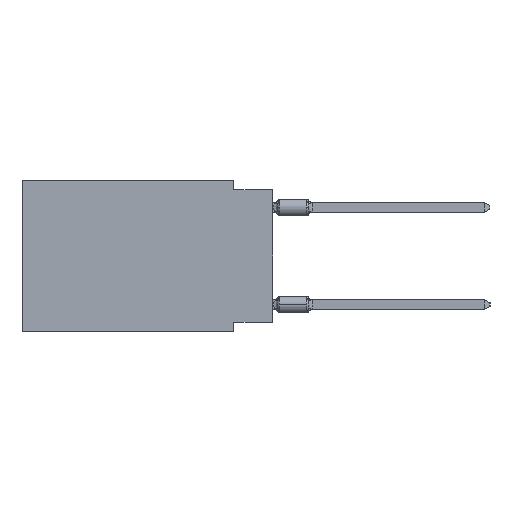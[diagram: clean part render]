
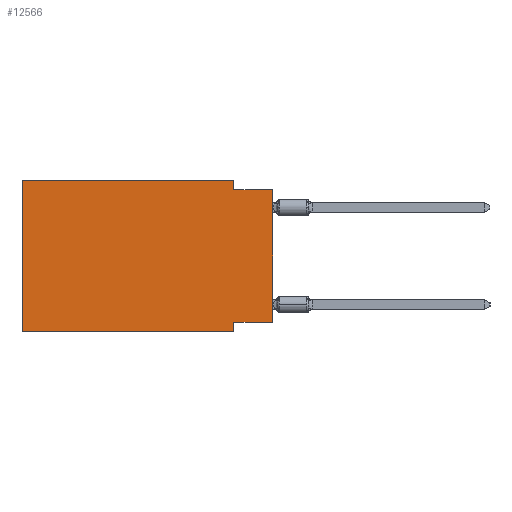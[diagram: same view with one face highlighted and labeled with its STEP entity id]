
A CAD part, left-side view. The second image highlights one B-rep face of the part: STEP entity #12566.
In plain terms, the highlighted planar face has unit normal (-1, 0, 0).
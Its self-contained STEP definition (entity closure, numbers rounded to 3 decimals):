
#699 = DIRECTION ( 'NONE',  ( 0., 0., 1. ) ) ;
#1057 = LINE ( 'NONE', #15567, #5075 ) ;
#2091 = CARTESIAN_POINT ( 'NONE',  ( 0., 2.54, -9.906 ) ) ;
#2407 = DIRECTION ( 'NONE',  ( 1., 0., 0. ) ) ;
#2442 = EDGE_CURVE ( 'NONE', #17567, #22266, #21646, .T. ) ;
#2515 = DIRECTION ( 'NONE',  ( 0., -1., 0. ) ) ;
#2831 = ORIENTED_EDGE ( 'NONE', *, *, #2442, .F. ) ;
#3285 = EDGE_LOOP ( 'NONE', ( #28138, #15857, #26342, #2831, #25457, #26435, #29695, #28562 ) ) ;
#3468 = VECTOR ( 'NONE', #11607, 1000. ) ;
#3684 = CARTESIAN_POINT ( 'NONE',  ( 0., 16.383, -9.906 ) ) ;
#4875 = FACE_OUTER_BOUND ( 'NONE', #3285, .T. ) ;
#5047 = PLANE ( 'NONE',  #10372 ) ;
#5075 = VECTOR ( 'NONE', #17880, 1000. ) ;
#5175 = CARTESIAN_POINT ( 'NONE',  ( 0., 16.383, 0. ) ) ;
#5462 = CARTESIAN_POINT ( 'NONE',  ( 0., 2.54, 0. ) ) ;
#6109 = LINE ( 'NONE', #26071, #17773 ) ;
#6618 = VERTEX_POINT ( 'NONE', #10996 ) ;
#6653 = CARTESIAN_POINT ( 'NONE',  ( 0., 0., 0. ) ) ;
#8192 = VECTOR ( 'NONE', #22129, 1000. ) ;
#8755 = VECTOR ( 'NONE', #25015, 1000. ) ;
#8970 = EDGE_CURVE ( 'NONE', #23673, #24792, #15040, .T. ) ;
#9190 = CARTESIAN_POINT ( 'NONE',  ( 0., 16.383, -9.906 ) ) ;
#9498 = VECTOR ( 'NONE', #2515, 1000. ) ;
#10372 = AXIS2_PLACEMENT_3D ( 'NONE', #29936, #2407, #15100 ) ;
#10996 = CARTESIAN_POINT ( 'NONE',  ( 0., 2.54, -9.271 ) ) ;
#11607 = DIRECTION ( 'NONE',  ( 0., 0., 1. ) ) ;
#12566 = ADVANCED_FACE ( 'NONE', ( #4875 ), #5047, .F. ) ;
#12947 = CARTESIAN_POINT ( 'NONE',  ( 0., 2.54, -0.635 ) ) ;
#13725 = EDGE_CURVE ( 'NONE', #6618, #31249, #6109, .T. ) ;
#15040 = LINE ( 'NONE', #25112, #9498 ) ;
#15100 = DIRECTION ( 'NONE',  ( 0., 0., -1. ) ) ;
#15471 = VERTEX_POINT ( 'NONE', #21390 ) ;
#15567 = CARTESIAN_POINT ( 'NONE',  ( 0., 2.54, 0. ) ) ;
#15857 = ORIENTED_EDGE ( 'NONE', *, *, #8970, .F. ) ;
#17340 = CARTESIAN_POINT ( 'NONE',  ( 0., 0., -0.635 ) ) ;
#17414 = CARTESIAN_POINT ( 'NONE',  ( 0., 0., -9.271 ) ) ;
#17567 = VERTEX_POINT ( 'NONE', #22792 ) ;
#17574 = LINE ( 'NONE', #17414, #8755 ) ;
#17773 = VECTOR ( 'NONE', #18135, 1000. ) ;
#17880 = DIRECTION ( 'NONE',  ( 0., 0., -1. ) ) ;
#18135 = DIRECTION ( 'NONE',  ( 0., 0., -1. ) ) ;
#18755 = LINE ( 'NONE', #9190, #25879 ) ;
#20800 = LINE ( 'NONE', #5175, #28158 ) ;
#21390 = CARTESIAN_POINT ( 'NONE',  ( 0., 0., -9.271 ) ) ;
#21646 = LINE ( 'NONE', #24619, #8192 ) ;
#21679 = EDGE_CURVE ( 'NONE', #30647, #31249, #18755, .T. ) ;
#21799 = LINE ( 'NONE', #6653, #3468 ) ;
#22129 = DIRECTION ( 'NONE',  ( 0., -1., 0. ) ) ;
#22266 = VERTEX_POINT ( 'NONE', #5462 ) ;
#22792 = CARTESIAN_POINT ( 'NONE',  ( 0., 16.383, 0. ) ) ;
#23629 = EDGE_CURVE ( 'NONE', #22266, #23673, #1057, .T. ) ;
#23673 = VERTEX_POINT ( 'NONE', #12947 ) ;
#23806 = EDGE_CURVE ( 'NONE', #15471, #24792, #21799, .T. ) ;
#24619 = CARTESIAN_POINT ( 'NONE',  ( 0., 16.383, 0. ) ) ;
#24792 = VERTEX_POINT ( 'NONE', #17340 ) ;
#25015 = DIRECTION ( 'NONE',  ( 0., 1., 0. ) ) ;
#25112 = CARTESIAN_POINT ( 'NONE',  ( 0., 0., -0.635 ) ) ;
#25457 = ORIENTED_EDGE ( 'NONE', *, *, #27444, .F. ) ;
#25879 = VECTOR ( 'NONE', #29142, 1000. ) ;
#26071 = CARTESIAN_POINT ( 'NONE',  ( 0., 2.54, -9.906 ) ) ;
#26342 = ORIENTED_EDGE ( 'NONE', *, *, #23629, .F. ) ;
#26435 = ORIENTED_EDGE ( 'NONE', *, *, #21679, .T. ) ;
#27444 = EDGE_CURVE ( 'NONE', #30647, #17567, #20800, .T. ) ;
#28138 = ORIENTED_EDGE ( 'NONE', *, *, #23806, .T. ) ;
#28158 = VECTOR ( 'NONE', #699, 1000. ) ;
#28562 = ORIENTED_EDGE ( 'NONE', *, *, #29939, .F. ) ;
#29142 = DIRECTION ( 'NONE',  ( 0., -1., 0. ) ) ;
#29695 = ORIENTED_EDGE ( 'NONE', *, *, #13725, .F. ) ;
#29936 = CARTESIAN_POINT ( 'NONE',  ( 0., 16.383, 0. ) ) ;
#29939 = EDGE_CURVE ( 'NONE', #15471, #6618, #17574, .T. ) ;
#30647 = VERTEX_POINT ( 'NONE', #3684 ) ;
#31249 = VERTEX_POINT ( 'NONE', #2091 ) ;
